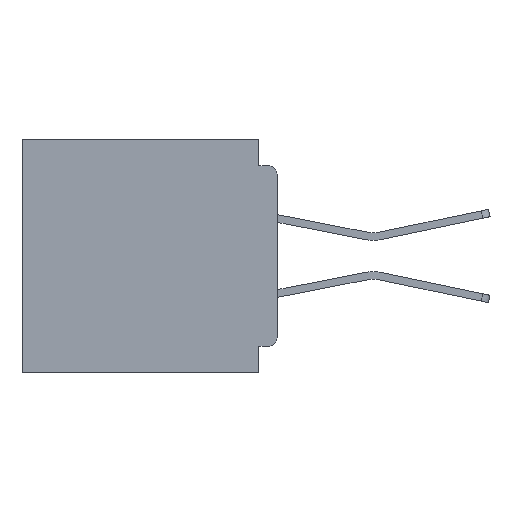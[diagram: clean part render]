
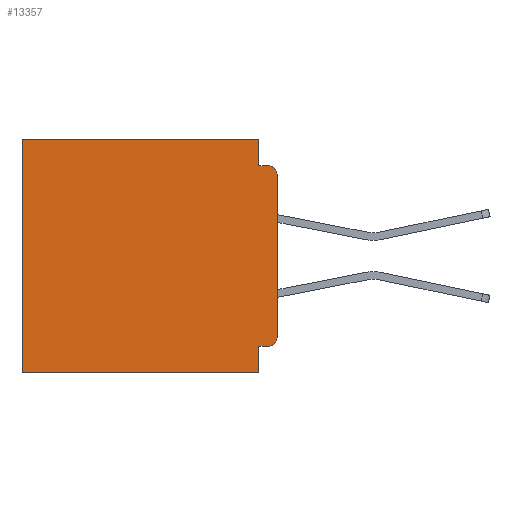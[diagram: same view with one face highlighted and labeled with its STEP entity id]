
A CAD part, left-side view. The second image highlights one B-rep face of the part: STEP entity #13357.
In plain terms, the highlighted planar face has unit normal (-1, 0, 0).
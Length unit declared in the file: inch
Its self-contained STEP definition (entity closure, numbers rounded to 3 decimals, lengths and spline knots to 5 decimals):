
#373 = VERTEX_POINT ( 'NONE', #38586 ) ;
#447 = DIRECTION ( 'NONE',  ( 0., 0., -1. ) ) ;
#726 = DIRECTION ( 'NONE',  ( 0., 0., -1. ) ) ;
#891 = LINE ( 'NONE', #11989, #8949 ) ;
#1545 = VECTOR ( 'NONE', #20163, 39.37008 ) ;
#1981 = EDGE_CURVE ( 'NONE', #19318, #24070, #11065, .T. ) ;
#2080 = VECTOR ( 'NONE', #24811, 39.37008 ) ;
#2215 = ORIENTED_EDGE ( 'NONE', *, *, #14162, .F. ) ;
#2503 = LINE ( 'NONE', #32022, #1545 ) ;
#2652 = CARTESIAN_POINT ( 'NONE',  ( 0.3, 0.031, -0.4 ) ) ;
#3037 = CIRCLE ( 'NONE', #20926, 0.015 ) ;
#3086 = CARTESIAN_POINT ( 'NONE',  ( 0.3, 0.015, -0.34 ) ) ;
#3657 = CARTESIAN_POINT ( 'NONE',  ( 0.3, 0., -0.4 ) ) ;
#3926 = VERTEX_POINT ( 'NONE', #35483 ) ;
#4166 = AXIS2_PLACEMENT_3D ( 'NONE', #3657, #18735, #726 ) ;
#4344 = CARTESIAN_POINT ( 'NONE',  ( 0.3, 0.437, -0.4 ) ) ;
#4501 = AXIS2_PLACEMENT_3D ( 'NONE', #3086, #24066, #6114 ) ;
#5759 = CARTESIAN_POINT ( 'NONE',  ( 0.3, 0.031, 0. ) ) ;
#6114 = DIRECTION ( 'NONE',  ( 0., 0., -1. ) ) ;
#6273 = CARTESIAN_POINT ( 'NONE',  ( 0.3, 0.015, -0.06 ) ) ;
#6299 = LINE ( 'NONE', #34961, #31068 ) ;
#6449 = VERTEX_POINT ( 'NONE', #29414 ) ;
#6456 = ORIENTED_EDGE ( 'NONE', *, *, #32734, .T. ) ;
#6903 = ORIENTED_EDGE ( 'NONE', *, *, #1981, .F. ) ;
#6937 = VERTEX_POINT ( 'NONE', #34478 ) ;
#7228 = VERTEX_POINT ( 'NONE', #9141 ) ;
#7775 = ORIENTED_EDGE ( 'NONE', *, *, #22656, .F. ) ;
#8340 = CIRCLE ( 'NONE', #4501, 0.015 ) ;
#8518 = ORIENTED_EDGE ( 'NONE', *, *, #38300, .T. ) ;
#8805 = DIRECTION ( 'NONE',  ( 0., 0., -1. ) ) ;
#8949 = VECTOR ( 'NONE', #26986, 39.37008 ) ;
#9141 = CARTESIAN_POINT ( 'NONE',  ( 0.3, 0., -0.34 ) ) ;
#9309 = DIRECTION ( 'NONE',  ( 0., 0., -1. ) ) ;
#9457 = LINE ( 'NONE', #5759, #24444 ) ;
#10071 = VERTEX_POINT ( 'NONE', #29978 ) ;
#10604 = LINE ( 'NONE', #34047, #33456 ) ;
#11065 = LINE ( 'NONE', #2652, #2080 ) ;
#11600 = EDGE_LOOP ( 'NONE', ( #28050, #8518, #2215, #19143, #6456, #31830, #7775, #6903, #33365, #28623 ) ) ;
#11989 = CARTESIAN_POINT ( 'NONE',  ( 0.3, 0., -0.4 ) ) ;
#13357 = ADVANCED_FACE ( 'NONE', ( #35322 ), #36582, .F. ) ;
#14162 = EDGE_CURVE ( 'NONE', #6449, #3926, #6299, .T. ) ;
#15835 = LINE ( 'NONE', #36302, #30731 ) ;
#16795 = EDGE_CURVE ( 'NONE', #6937, #6449, #9457, .T. ) ;
#17134 = DIRECTION ( 'NONE',  ( 0., -1., 0. ) ) ;
#18735 = DIRECTION ( 'NONE',  ( 1., 0., 0. ) ) ;
#18825 = CARTESIAN_POINT ( 'NONE',  ( 0.3, 0.437, -0.4 ) ) ;
#19143 = ORIENTED_EDGE ( 'NONE', *, *, #16795, .F. ) ;
#19318 = VERTEX_POINT ( 'NONE', #28286 ) ;
#20100 = VECTOR ( 'NONE', #24855, 39.37008 ) ;
#20163 = DIRECTION ( 'NONE',  ( 0., 1., 0. ) ) ;
#20926 = AXIS2_PLACEMENT_3D ( 'NONE', #6273, #27216, #9309 ) ;
#21040 = VERTEX_POINT ( 'NONE', #22536 ) ;
#22536 = CARTESIAN_POINT ( 'NONE',  ( 0.3, 0., -0.06 ) ) ;
#22656 = EDGE_CURVE ( 'NONE', #24070, #25208, #891, .T. ) ;
#24066 = DIRECTION ( 'NONE',  ( -1., 0., 0. ) ) ;
#24070 = VERTEX_POINT ( 'NONE', #37594 ) ;
#24444 = VECTOR ( 'NONE', #8805, 39.37008 ) ;
#24811 = DIRECTION ( 'NONE',  ( 0., 0., -1. ) ) ;
#24855 = DIRECTION ( 'NONE',  ( 0., 0., -1. ) ) ;
#25208 = VERTEX_POINT ( 'NONE', #4344 ) ;
#25258 = LINE ( 'NONE', #18825, #20100 ) ;
#26986 = DIRECTION ( 'NONE',  ( 0., 1., 0. ) ) ;
#27216 = DIRECTION ( 'NONE',  ( -1., 0., 0. ) ) ;
#28050 = ORIENTED_EDGE ( 'NONE', *, *, #31908, .F. ) ;
#28286 = CARTESIAN_POINT ( 'NONE',  ( 0.3, 0.031, -0.355 ) ) ;
#28623 = ORIENTED_EDGE ( 'NONE', *, *, #31665, .T. ) ;
#29414 = CARTESIAN_POINT ( 'NONE',  ( 0.3, 0.031, -0.045 ) ) ;
#29978 = CARTESIAN_POINT ( 'NONE',  ( 0.3, 0.015, -0.355 ) ) ;
#30731 = VECTOR ( 'NONE', #447, 39.37008 ) ;
#31068 = VECTOR ( 'NONE', #17134, 39.37008 ) ;
#31665 = EDGE_CURVE ( 'NONE', #10071, #7228, #8340, .T. ) ;
#31830 = ORIENTED_EDGE ( 'NONE', *, *, #35993, .T. ) ;
#31908 = EDGE_CURVE ( 'NONE', #21040, #7228, #15835, .T. ) ;
#32022 = CARTESIAN_POINT ( 'NONE',  ( 0.3, 0., -0.355 ) ) ;
#32734 = EDGE_CURVE ( 'NONE', #6937, #373, #10604, .T. ) ;
#33365 = ORIENTED_EDGE ( 'NONE', *, *, #33592, .F. ) ;
#33456 = VECTOR ( 'NONE', #34171, 39.37008 ) ;
#33592 = EDGE_CURVE ( 'NONE', #10071, #19318, #2503, .T. ) ;
#34047 = CARTESIAN_POINT ( 'NONE',  ( 0.3, 0., 0. ) ) ;
#34171 = DIRECTION ( 'NONE',  ( 0., 1., 0. ) ) ;
#34478 = CARTESIAN_POINT ( 'NONE',  ( 0.3, 0.031, 0. ) ) ;
#34961 = CARTESIAN_POINT ( 'NONE',  ( 0.3, 0., -0.045 ) ) ;
#35322 = FACE_OUTER_BOUND ( 'NONE', #11600, .T. ) ;
#35483 = CARTESIAN_POINT ( 'NONE',  ( 0.3, 0.015, -0.045 ) ) ;
#35993 = EDGE_CURVE ( 'NONE', #373, #25208, #25258, .T. ) ;
#36302 = CARTESIAN_POINT ( 'NONE',  ( 0.3, 0., -0.4 ) ) ;
#36582 = PLANE ( 'NONE',  #4166 ) ;
#37594 = CARTESIAN_POINT ( 'NONE',  ( 0.3, 0.031, -0.4 ) ) ;
#38300 = EDGE_CURVE ( 'NONE', #21040, #3926, #3037, .T. ) ;
#38586 = CARTESIAN_POINT ( 'NONE',  ( 0.3, 0.437, 0. ) ) ;
